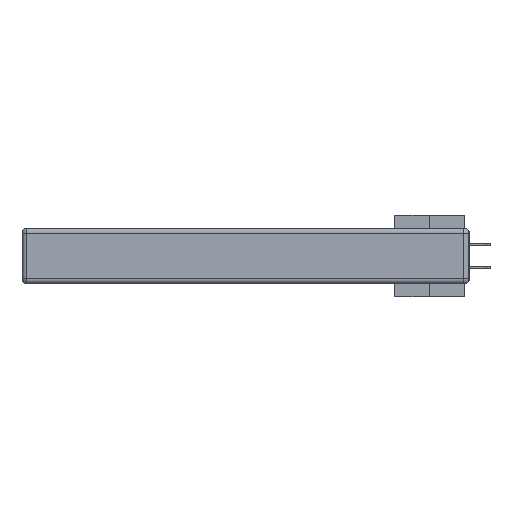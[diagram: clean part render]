
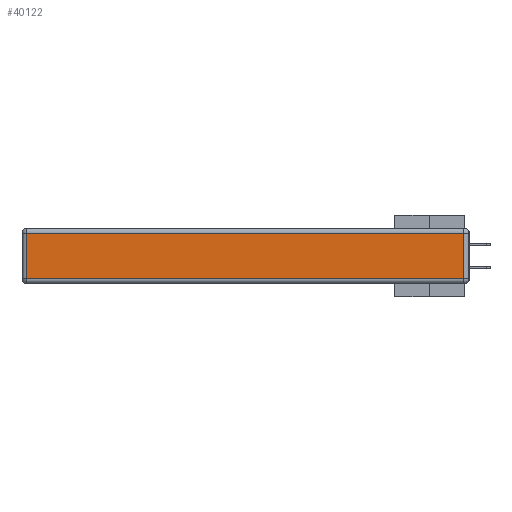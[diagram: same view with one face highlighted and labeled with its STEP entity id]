
A CAD part, left-side view. The second image highlights one B-rep face of the part: STEP entity #40122.
In plain terms, the highlighted planar face has unit normal (-1, 0, 0).
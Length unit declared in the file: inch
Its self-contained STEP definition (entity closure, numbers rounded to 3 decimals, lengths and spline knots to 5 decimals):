
#707 = VERTEX_POINT ( 'NONE', #14160 ) ;
#3818 = VERTEX_POINT ( 'NONE', #10741 ) ;
#5738 = LINE ( 'NONE', #23489, #41752 ) ;
#5946 = EDGE_CURVE ( 'NONE', #35443, #3818, #18293, .T. ) ;
#8182 = DIRECTION ( 'NONE',  ( 0., -1., 0. ) ) ;
#10741 = CARTESIAN_POINT ( 'NONE',  ( 0., 0.03, -0.03 ) ) ;
#14127 = LINE ( 'NONE', #27286, #36556 ) ;
#14160 = CARTESIAN_POINT ( 'NONE',  ( 0., 2.72, -0.03 ) ) ;
#14711 = ORIENTED_EDGE ( 'NONE', *, *, #29424, .T. ) ;
#16684 = PLANE ( 'NONE',  #44140 ) ;
#17113 = CARTESIAN_POINT ( 'NONE',  ( 0., 0., -0.343 ) ) ;
#17832 = EDGE_CURVE ( 'NONE', #31735, #35443, #42078, .T. ) ;
#18293 = LINE ( 'NONE', #31981, #29795 ) ;
#20409 = DIRECTION ( 'NONE',  ( 0., 0., -1. ) ) ;
#22984 = ORIENTED_EDGE ( 'NONE', *, *, #38662, .T. ) ;
#23489 = CARTESIAN_POINT ( 'NONE',  ( 0., 2.72, -0.343 ) ) ;
#23614 = ORIENTED_EDGE ( 'NONE', *, *, #17832, .T. ) ;
#27286 = CARTESIAN_POINT ( 'NONE',  ( 0., 2.75, -0.03 ) ) ;
#27379 = DIRECTION ( 'NONE',  ( -1., 0., 0. ) ) ;
#27933 = VECTOR ( 'NONE', #8182, 39.37008 ) ;
#27941 = EDGE_LOOP ( 'NONE', ( #23614, #31313, #22984, #14711 ) ) ;
#28800 = CARTESIAN_POINT ( 'NONE',  ( 0., 0., -0.313 ) ) ;
#29318 = CARTESIAN_POINT ( 'NONE',  ( 0., 0.03, -0.313 ) ) ;
#29424 = EDGE_CURVE ( 'NONE', #707, #31735, #5738, .T. ) ;
#29795 = VECTOR ( 'NONE', #33058, 39.37008 ) ;
#31313 = ORIENTED_EDGE ( 'NONE', *, *, #5946, .T. ) ;
#31735 = VERTEX_POINT ( 'NONE', #41605 ) ;
#31981 = CARTESIAN_POINT ( 'NONE',  ( 0., 0.03, -0.343 ) ) ;
#33058 = DIRECTION ( 'NONE',  ( 0., 0., 1. ) ) ;
#34195 = FACE_OUTER_BOUND ( 'NONE', #27941, .T. ) ;
#34810 = DIRECTION ( 'NONE',  ( 0., 0., 1. ) ) ;
#35443 = VERTEX_POINT ( 'NONE', #29318 ) ;
#36556 = VECTOR ( 'NONE', #44664, 39.37008 ) ;
#38662 = EDGE_CURVE ( 'NONE', #3818, #707, #14127, .T. ) ;
#40122 = ADVANCED_FACE ( 'NONE', ( #34195 ), #16684, .T. ) ;
#41605 = CARTESIAN_POINT ( 'NONE',  ( 0., 2.72, -0.313 ) ) ;
#41752 = VECTOR ( 'NONE', #20409, 39.37008 ) ;
#42078 = LINE ( 'NONE', #28800, #27933 ) ;
#44140 = AXIS2_PLACEMENT_3D ( 'NONE', #17113, #27379, #34810 ) ;
#44664 = DIRECTION ( 'NONE',  ( 0., 1., 0. ) ) ;
